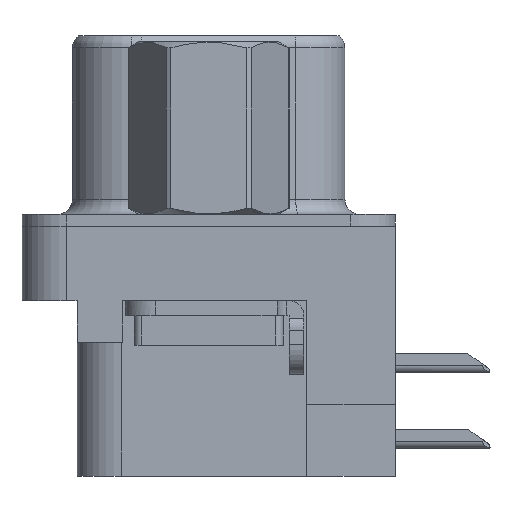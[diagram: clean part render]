
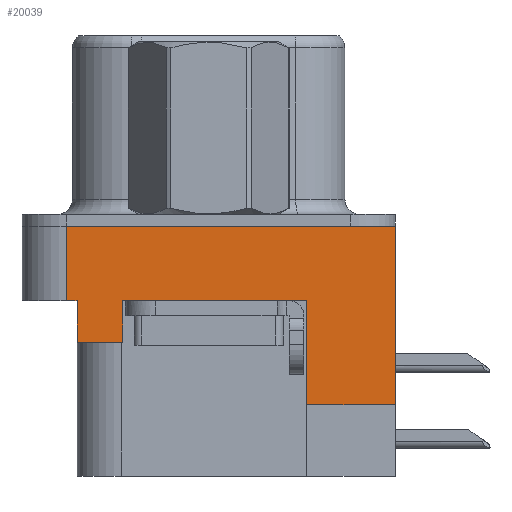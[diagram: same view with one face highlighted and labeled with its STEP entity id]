
A CAD part, left-side view. The second image highlights one B-rep face of the part: STEP entity #20039.
In plain terms, the highlighted planar face has unit normal (-1, 0, 0).
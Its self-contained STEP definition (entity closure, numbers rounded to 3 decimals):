
#698 = VERTEX_POINT ( 'NONE', #4368 ) ;
#1032 = DIRECTION ( 'NONE',  ( 0., -1., 0. ) ) ;
#1066 = LINE ( 'NONE', #12071, #19123 ) ;
#1562 = EDGE_CURVE ( 'NONE', #6488, #1965, #4162, .T. ) ;
#1911 = EDGE_LOOP ( 'NONE', ( #21652, #12095, #2453, #19615, #7271, #22602, #22425, #14987, #10741, #19829 ) ) ;
#1965 = VERTEX_POINT ( 'NONE', #22401 ) ;
#2032 = VERTEX_POINT ( 'NONE', #16610 ) ;
#2453 = ORIENTED_EDGE ( 'NONE', *, *, #23141, .F. ) ;
#2594 = DIRECTION ( 'NONE',  ( 0., -1., 0. ) ) ;
#2645 = CARTESIAN_POINT ( 'NONE',  ( -2.935, -6.275, -6. ) ) ;
#2748 = CARTESIAN_POINT ( 'NONE',  ( -2.935, 2.895, -3.9 ) ) ;
#2781 = EDGE_CURVE ( 'NONE', #698, #8090, #17380, .T. ) ;
#3193 = DIRECTION ( 'NONE',  ( 0., 0., 1. ) ) ;
#3582 = LINE ( 'NONE', #22350, #7019 ) ;
#3793 = EDGE_CURVE ( 'NONE', #19138, #6488, #10003, .T. ) ;
#4162 = LINE ( 'NONE', #11711, #18542 ) ;
#4338 = CARTESIAN_POINT ( 'NONE',  ( -2.935, -6.275, -2.5 ) ) ;
#4368 = CARTESIAN_POINT ( 'NONE',  ( -2.935, 4.775, -2.5 ) ) ;
#4429 = EDGE_CURVE ( 'NONE', #19138, #21785, #4629, .T. ) ;
#4570 = EDGE_CURVE ( 'NONE', #9784, #2032, #16167, .T. ) ;
#4629 = LINE ( 'NONE', #4338, #8846 ) ;
#4676 = LINE ( 'NONE', #17543, #9442 ) ;
#5761 = VECTOR ( 'NONE', #5860, 1000. ) ;
#5860 = DIRECTION ( 'NONE',  ( 0., 1., 0. ) ) ;
#6472 = DIRECTION ( 'NONE',  ( 0., 0., 1. ) ) ;
#6488 = VERTEX_POINT ( 'NONE', #18920 ) ;
#6648 = DIRECTION ( 'NONE',  ( 0., 1., 0. ) ) ;
#7011 = EDGE_CURVE ( 'NONE', #17267, #1965, #4676, .T. ) ;
#7019 = VECTOR ( 'NONE', #2594, 1000. ) ;
#7271 = ORIENTED_EDGE ( 'NONE', *, *, #12437, .T. ) ;
#8090 = VERTEX_POINT ( 'NONE', #20287 ) ;
#8647 = FACE_OUTER_BOUND ( 'NONE', #1911, .T. ) ;
#8846 = VECTOR ( 'NONE', #13299, 1000. ) ;
#8863 = CARTESIAN_POINT ( 'NONE',  ( -2.935, -6.275, -2.5 ) ) ;
#9442 = VECTOR ( 'NONE', #13991, 1000. ) ;
#9784 = VERTEX_POINT ( 'NONE', #20869 ) ;
#10003 = LINE ( 'NONE', #14830, #5761 ) ;
#10107 = CARTESIAN_POINT ( 'NONE',  ( -2.935, 4.425, -3.9 ) ) ;
#10206 = VERTEX_POINT ( 'NONE', #14050 ) ;
#10619 = LINE ( 'NONE', #2748, #19624 ) ;
#10684 = DIRECTION ( 'NONE',  ( -1., 0., 0. ) ) ;
#10741 = ORIENTED_EDGE ( 'NONE', *, *, #7011, .T. ) ;
#11711 = CARTESIAN_POINT ( 'NONE',  ( -2.935, -3.295, -8.4 ) ) ;
#11841 = CARTESIAN_POINT ( 'NONE',  ( -2.935, -6.275, 0. ) ) ;
#12071 = CARTESIAN_POINT ( 'NONE',  ( -2.935, 4.425, -3.9 ) ) ;
#12095 = ORIENTED_EDGE ( 'NONE', *, *, #4429, .T. ) ;
#12437 = EDGE_CURVE ( 'NONE', #698, #2032, #3582, .T. ) ;
#12518 = CARTESIAN_POINT ( 'NONE',  ( -2.935, 2.895, -2.5 ) ) ;
#13299 = DIRECTION ( 'NONE',  ( 0., 0., 1. ) ) ;
#13657 = EDGE_CURVE ( 'NONE', #10206, #17267, #10619, .T. ) ;
#13991 = DIRECTION ( 'NONE',  ( 0., -1., 0. ) ) ;
#14050 = CARTESIAN_POINT ( 'NONE',  ( -2.935, 2.895, -3.9 ) ) ;
#14830 = CARTESIAN_POINT ( 'NONE',  ( -2.935, -6.495, -6. ) ) ;
#14987 = ORIENTED_EDGE ( 'NONE', *, *, #13657, .T. ) ;
#15239 = LINE ( 'NONE', #11841, #20020 ) ;
#16167 = LINE ( 'NONE', #10107, #20358 ) ;
#16256 = VECTOR ( 'NONE', #16564, 1000. ) ;
#16564 = DIRECTION ( 'NONE',  ( 0., 0., 1. ) ) ;
#16610 = CARTESIAN_POINT ( 'NONE',  ( -2.935, 4.425, -2.5 ) ) ;
#17267 = VERTEX_POINT ( 'NONE', #12518 ) ;
#17380 = LINE ( 'NONE', #18288, #16256 ) ;
#17543 = CARTESIAN_POINT ( 'NONE',  ( -2.935, -6.275, -2.5 ) ) ;
#18288 = CARTESIAN_POINT ( 'NONE',  ( -2.935, 4.775, -2.5 ) ) ;
#18542 = VECTOR ( 'NONE', #3193, 1000. ) ;
#18576 = EDGE_CURVE ( 'NONE', #10206, #9784, #1066, .T. ) ;
#18920 = CARTESIAN_POINT ( 'NONE',  ( -2.935, -3.295, -6. ) ) ;
#19123 = VECTOR ( 'NONE', #6648, 1000. ) ;
#19138 = VERTEX_POINT ( 'NONE', #2645 ) ;
#19615 = ORIENTED_EDGE ( 'NONE', *, *, #2781, .F. ) ;
#19624 = VECTOR ( 'NONE', #22660, 1000. ) ;
#19829 = ORIENTED_EDGE ( 'NONE', *, *, #1562, .F. ) ;
#20020 = VECTOR ( 'NONE', #1032, 1000. ) ;
#20039 = ADVANCED_FACE ( 'NONE', ( #8647 ), #21424, .T. ) ;
#20287 = CARTESIAN_POINT ( 'NONE',  ( -2.935, 4.775, 0. ) ) ;
#20358 = VECTOR ( 'NONE', #6472, 1000. ) ;
#20869 = CARTESIAN_POINT ( 'NONE',  ( -2.935, 4.425, -3.9 ) ) ;
#21424 = PLANE ( 'NONE',  #21655 ) ;
#21652 = ORIENTED_EDGE ( 'NONE', *, *, #3793, .F. ) ;
#21655 = AXIS2_PLACEMENT_3D ( 'NONE', #8863, #10684, #23232 ) ;
#21785 = VERTEX_POINT ( 'NONE', #22244 ) ;
#22244 = CARTESIAN_POINT ( 'NONE',  ( -2.935, -6.275, 0. ) ) ;
#22350 = CARTESIAN_POINT ( 'NONE',  ( -2.935, -6.275, -2.5 ) ) ;
#22401 = CARTESIAN_POINT ( 'NONE',  ( -2.935, -3.295, -2.5 ) ) ;
#22425 = ORIENTED_EDGE ( 'NONE', *, *, #18576, .F. ) ;
#22602 = ORIENTED_EDGE ( 'NONE', *, *, #4570, .F. ) ;
#22660 = DIRECTION ( 'NONE',  ( 0., 0., 1. ) ) ;
#23141 = EDGE_CURVE ( 'NONE', #8090, #21785, #15239, .T. ) ;
#23232 = DIRECTION ( 'NONE',  ( 0., 0., 1. ) ) ;
